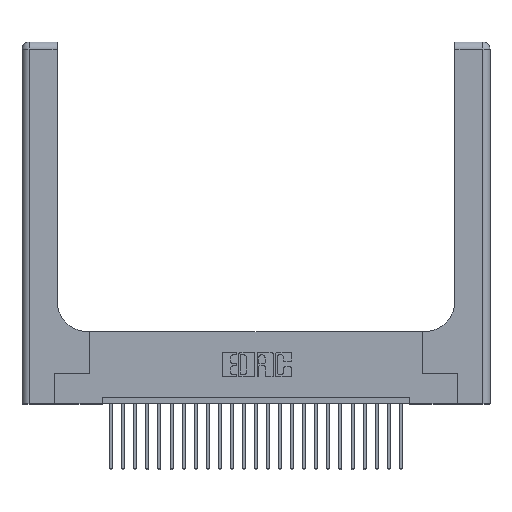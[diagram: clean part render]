
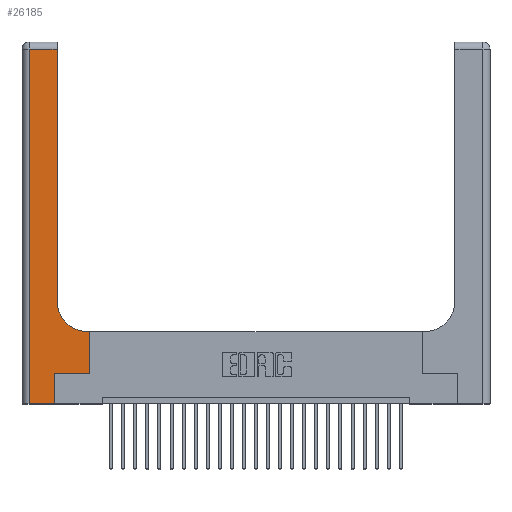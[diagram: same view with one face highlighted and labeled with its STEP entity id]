
A CAD part, top view. The second image highlights one B-rep face of the part: STEP entity #26185.
In plain terms, the highlighted planar face has unit normal (0, 0, 1).
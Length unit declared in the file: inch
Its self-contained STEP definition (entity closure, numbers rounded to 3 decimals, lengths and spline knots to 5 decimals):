
#577 = EDGE_CURVE ( 'NONE', #10453, #17578, #25117, .T. ) ;
#822 = EDGE_CURVE ( 'NONE', #17578, #20609, #23786, .T. ) ;
#874 = VECTOR ( 'NONE', #23497, 39.37008 ) ;
#1029 = EDGE_CURVE ( 'NONE', #17350, #20112, #3795, .T. ) ;
#2152 = ORIENTED_EDGE ( 'NONE', *, *, #1029, .T. ) ;
#2296 = VECTOR ( 'NONE', #16658, 39.37008 ) ;
#2333 = EDGE_CURVE ( 'NONE', #20112, #11162, #11929, .T. ) ;
#2721 = ORIENTED_EDGE ( 'NONE', *, *, #2333, .T. ) ;
#2945 = LINE ( 'NONE', #22692, #2296 ) ;
#3795 = LINE ( 'NONE', #23283, #23448 ) ;
#4326 = ORIENTED_EDGE ( 'NONE', *, *, #22502, .T. ) ;
#5043 = FACE_OUTER_BOUND ( 'NONE', #25316, .T. ) ;
#5392 = VECTOR ( 'NONE', #14805, 39.37008 ) ;
#5773 = DIRECTION ( 'NONE',  ( 0., 0., -1. ) ) ;
#7178 = LINE ( 'NONE', #9192, #21446 ) ;
#7399 = CARTESIAN_POINT ( 'NONE',  ( 0.5585, 0.25, 0.37 ) ) ;
#7623 = CARTESIAN_POINT ( 'NONE',  ( 0.269, 0.25, 0.37 ) ) ;
#7904 = ORIENTED_EDGE ( 'NONE', *, *, #822, .T. ) ;
#8359 = ORIENTED_EDGE ( 'NONE', *, *, #21641, .T. ) ;
#9005 = DIRECTION ( 'NONE',  ( 0., 1., 0. ) ) ;
#9192 = CARTESIAN_POINT ( 'NONE',  ( 0.06, 3., 0.37 ) ) ;
#9884 = CARTESIAN_POINT ( 'NONE',  ( 0., 3., 0.37 ) ) ;
#9900 = ORIENTED_EDGE ( 'NONE', *, *, #18348, .T. ) ;
#9939 = CARTESIAN_POINT ( 'NONE',  ( 0.2915, 0.85, 0.37 ) ) ;
#10372 = LINE ( 'NONE', #13950, #16079 ) ;
#10453 = VERTEX_POINT ( 'NONE', #9939 ) ;
#10665 = VERTEX_POINT ( 'NONE', #12693 ) ;
#10743 = CARTESIAN_POINT ( 'NONE',  ( 0.2915, 3., 0.37 ) ) ;
#11162 = VERTEX_POINT ( 'NONE', #7399 ) ;
#11518 = EDGE_CURVE ( 'NONE', #10665, #17350, #2945, .T. ) ;
#11566 = CARTESIAN_POINT ( 'NONE',  ( 0.269, 0.25, 0.37 ) ) ;
#11929 = LINE ( 'NONE', #11566, #874 ) ;
#12024 = CARTESIAN_POINT ( 'NONE',  ( 0.269, 0., 0.37 ) ) ;
#12073 = PLANE ( 'NONE',  #21535 ) ;
#12345 = VECTOR ( 'NONE', #17455, 39.37008 ) ;
#12693 = CARTESIAN_POINT ( 'NONE',  ( 0.06, 0., 0.37 ) ) ;
#12891 = EDGE_CURVE ( 'NONE', #11162, #24701, #10372, .T. ) ;
#13017 = VECTOR ( 'NONE', #21734, 39.37008 ) ;
#13858 = CARTESIAN_POINT ( 'NONE',  ( 0.2915, 2.94, 0.37 ) ) ;
#13950 = CARTESIAN_POINT ( 'NONE',  ( 0.5585, 0.25, 0.37 ) ) ;
#13986 = CARTESIAN_POINT ( 'NONE',  ( 0., 2.94, 0.37 ) ) ;
#14805 = DIRECTION ( 'NONE',  ( -1., 0., 0. ) ) ;
#15321 = ORIENTED_EDGE ( 'NONE', *, *, #11518, .T. ) ;
#15356 = CIRCLE ( 'NONE', #17903, 0.25 ) ;
#15459 = CARTESIAN_POINT ( 'NONE',  ( 0.5415, 0.6, 0.37 ) ) ;
#15883 = DIRECTION ( 'NONE',  ( 0., 1., 0. ) ) ;
#15988 = DIRECTION ( 'NONE',  ( 0., 0., -1. ) ) ;
#16079 = VECTOR ( 'NONE', #15883, 39.37008 ) ;
#16658 = DIRECTION ( 'NONE',  ( 1., 0., 0. ) ) ;
#16962 = VERTEX_POINT ( 'NONE', #15459 ) ;
#17350 = VERTEX_POINT ( 'NONE', #12024 ) ;
#17455 = DIRECTION ( 'NONE',  ( 0., 1., 0. ) ) ;
#17459 = LINE ( 'NONE', #25424, #13017 ) ;
#17578 = VERTEX_POINT ( 'NONE', #13858 ) ;
#17903 = AXIS2_PLACEMENT_3D ( 'NONE', #20272, #5773, #18168 ) ;
#18168 = DIRECTION ( 'NONE',  ( 1., 0., 0. ) ) ;
#18348 = EDGE_CURVE ( 'NONE', #24701, #16962, #17459, .T. ) ;
#18456 = ORIENTED_EDGE ( 'NONE', *, *, #12891, .T. ) ;
#20112 = VERTEX_POINT ( 'NONE', #7623 ) ;
#20272 = CARTESIAN_POINT ( 'NONE',  ( 0.5415, 0.85, 0.37 ) ) ;
#20609 = VERTEX_POINT ( 'NONE', #23493 ) ;
#21446 = VECTOR ( 'NONE', #25443, 39.37008 ) ;
#21535 = AXIS2_PLACEMENT_3D ( 'NONE', #9884, #15988, #22213 ) ;
#21641 = EDGE_CURVE ( 'NONE', #20609, #10665, #7178, .T. ) ;
#21734 = DIRECTION ( 'NONE',  ( -1., 0., 0. ) ) ;
#22213 = DIRECTION ( 'NONE',  ( -1., 0., 0. ) ) ;
#22400 = ORIENTED_EDGE ( 'NONE', *, *, #577, .T. ) ;
#22502 = EDGE_CURVE ( 'NONE', #16962, #10453, #15356, .T. ) ;
#22692 = CARTESIAN_POINT ( 'NONE',  ( 0., 0., 0.37 ) ) ;
#23283 = CARTESIAN_POINT ( 'NONE',  ( 0.269, 0., 0.37 ) ) ;
#23448 = VECTOR ( 'NONE', #9005, 39.37008 ) ;
#23493 = CARTESIAN_POINT ( 'NONE',  ( 0.06, 2.94, 0.37 ) ) ;
#23497 = DIRECTION ( 'NONE',  ( 1., 0., 0. ) ) ;
#23786 = LINE ( 'NONE', #13986, #5392 ) ;
#24701 = VERTEX_POINT ( 'NONE', #25344 ) ;
#25117 = LINE ( 'NONE', #10743, #12345 ) ;
#25316 = EDGE_LOOP ( 'NONE', ( #22400, #7904, #8359, #15321, #2152, #2721, #18456, #9900, #4326 ) ) ;
#25344 = CARTESIAN_POINT ( 'NONE',  ( 0.5585, 0.6, 0.37 ) ) ;
#25424 = CARTESIAN_POINT ( 'NONE',  ( 0.2915, 0.6, 0.37 ) ) ;
#25443 = DIRECTION ( 'NONE',  ( 0., -1., 0. ) ) ;
#26185 = ADVANCED_FACE ( 'NONE', ( #5043 ), #12073, .F. ) ;
